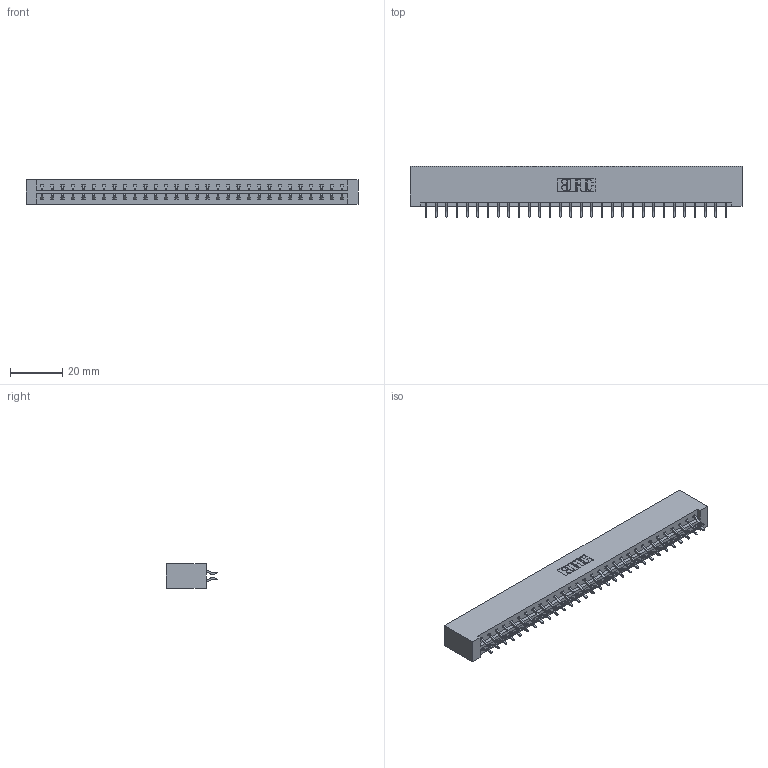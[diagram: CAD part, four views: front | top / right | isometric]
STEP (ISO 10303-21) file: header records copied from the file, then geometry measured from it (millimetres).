
FILE_DESCRIPTION (( 'STEP AP203' ), '1' );
FILE_NAME ('833-060-556-201.STEP', '2020-06-05T04:30:33', ( '' ), ( '' ), 'SwSTEP 2.0', 'SolidWorks 2020', '' );
FILE_SCHEMA (( 'CONFIG_CONTROL_DESIGN' ));
Length unit declared in the file: inch
Products named in the file (3): 833 Part_Lugless; 345-292-001_556 Tail; 833-060-556-201
Assembly tree (61 placements, depth 2):
  833-060-556-201
    833 Part_Lugless
    345-292-001_556 Tail  x60
Bounding box: 127.13 x 19.57 x 9.4 mm (x, y, z)
Volume: 13496.6 mm3; surface area: 15792.5 mm2
Topology: 61 solids, 61 shells, 3586 faces, 10667 edges, 7030 vertices
Faces by surface type: plane 2466, cylinder 1120
Entity records: 20795 total; most frequent: CARTESIAN_POINT 3474, ORIENTED_EDGE 3398, DIRECTION 2971, EDGE_CURVE 1699, VECTOR 1571, LINE 1571, VERTEX_POINT 1130, AXIS2_PLACEMENT_3D 700
